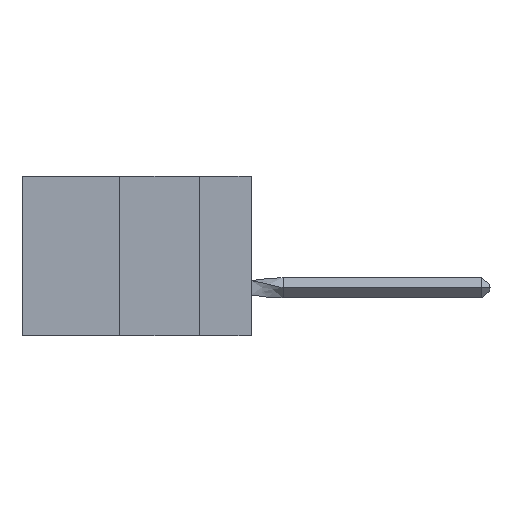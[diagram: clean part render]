
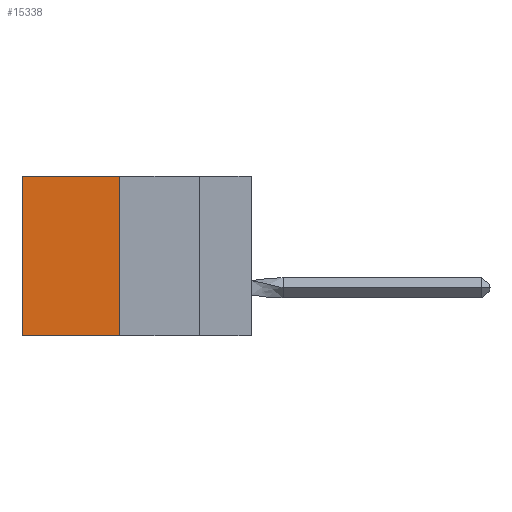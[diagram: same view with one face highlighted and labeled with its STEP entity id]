
A CAD part, left-side view. The second image highlights one B-rep face of the part: STEP entity #15338.
In plain terms, the highlighted planar face has unit normal (-1, 0, 0).
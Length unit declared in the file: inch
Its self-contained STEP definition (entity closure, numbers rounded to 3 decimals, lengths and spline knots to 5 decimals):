
#250 = DIRECTION ( 'NONE',  ( 0., 1., 0. ) ) ;
#522 = EDGE_CURVE ( 'NONE', #10892, #7623, #6840, .T. ) ;
#1222 = DIRECTION ( 'NONE',  ( 1., 0., 0. ) ) ;
#1517 = CARTESIAN_POINT ( 'NONE',  ( 0.305, 0.413, -0.5 ) ) ;
#2182 = CARTESIAN_POINT ( 'NONE',  ( 0.305, 0.72, -0.5 ) ) ;
#3437 = VECTOR ( 'NONE', #11057, 39.37008 ) ;
#3725 = EDGE_CURVE ( 'NONE', #10892, #15005, #12282, .T. ) ;
#3952 = VECTOR ( 'NONE', #5529, 39.37008 ) ;
#4083 = DIRECTION ( 'NONE',  ( 0., 0., -1. ) ) ;
#4288 = FACE_OUTER_BOUND ( 'NONE', #10660, .T. ) ;
#5529 = DIRECTION ( 'NONE',  ( 0., 1., 0. ) ) ;
#5761 = CARTESIAN_POINT ( 'NONE',  ( 0.305, 0.413, 0. ) ) ;
#5851 = VECTOR ( 'NONE', #4083, 39.37008 ) ;
#5895 = VERTEX_POINT ( 'NONE', #9822 ) ;
#6043 = EDGE_CURVE ( 'NONE', #7623, #5895, #13209, .T. ) ;
#6050 = PLANE ( 'NONE',  #11534 ) ;
#6279 = CARTESIAN_POINT ( 'NONE',  ( 0.305, 0.413, -0.5 ) ) ;
#6840 = LINE ( 'NONE', #1517, #5851 ) ;
#6939 = CARTESIAN_POINT ( 'NONE',  ( 0.305, 0.72, 0. ) ) ;
#7623 = VERTEX_POINT ( 'NONE', #10742 ) ;
#9082 = DIRECTION ( 'NONE',  ( 0., 0., -1. ) ) ;
#9147 = ORIENTED_EDGE ( 'NONE', *, *, #3725, .T. ) ;
#9671 = VECTOR ( 'NONE', #250, 39.37008 ) ;
#9822 = CARTESIAN_POINT ( 'NONE',  ( 0.305, 0.72, -0.5 ) ) ;
#9865 = EDGE_CURVE ( 'NONE', #15005, #5895, #13887, .T. ) ;
#10660 = EDGE_LOOP ( 'NONE', ( #12069, #15796, #13482, #9147 ) ) ;
#10742 = CARTESIAN_POINT ( 'NONE',  ( 0.305, 0.413, -0.5 ) ) ;
#10892 = VERTEX_POINT ( 'NONE', #5761 ) ;
#11057 = DIRECTION ( 'NONE',  ( 0., 0., -1. ) ) ;
#11534 = AXIS2_PLACEMENT_3D ( 'NONE', #6279, #1222, #9082 ) ;
#11694 = CARTESIAN_POINT ( 'NONE',  ( 0.305, 0.413, -0.5 ) ) ;
#12069 = ORIENTED_EDGE ( 'NONE', *, *, #9865, .T. ) ;
#12282 = LINE ( 'NONE', #14552, #3952 ) ;
#13209 = LINE ( 'NONE', #11694, #9671 ) ;
#13482 = ORIENTED_EDGE ( 'NONE', *, *, #522, .F. ) ;
#13887 = LINE ( 'NONE', #2182, #3437 ) ;
#14552 = CARTESIAN_POINT ( 'NONE',  ( 0.305, 0.413, 0. ) ) ;
#15005 = VERTEX_POINT ( 'NONE', #6939 ) ;
#15338 = ADVANCED_FACE ( 'NONE', ( #4288 ), #6050, .F. ) ;
#15796 = ORIENTED_EDGE ( 'NONE', *, *, #6043, .F. ) ;
